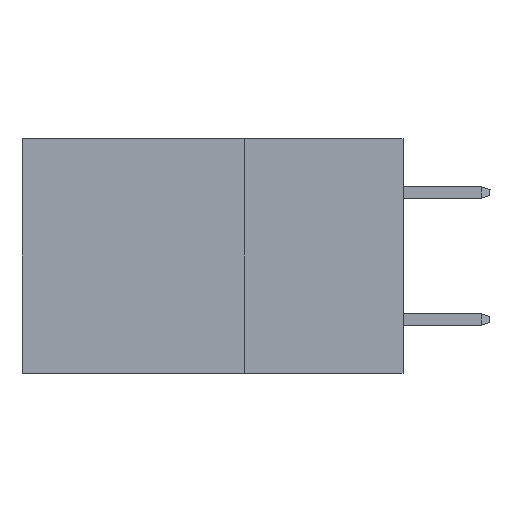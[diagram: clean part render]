
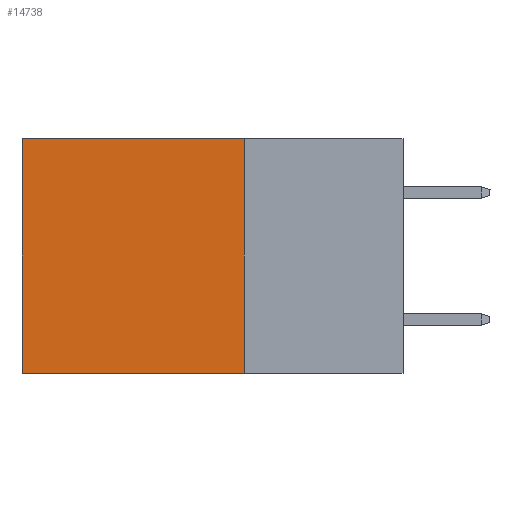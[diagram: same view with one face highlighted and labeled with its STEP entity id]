
A CAD part, left-side view. The second image highlights one B-rep face of the part: STEP entity #14738.
In plain terms, the highlighted planar face has unit normal (-1, 0, 0).
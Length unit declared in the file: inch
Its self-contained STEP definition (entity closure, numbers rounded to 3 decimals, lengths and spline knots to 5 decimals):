
#822 = EDGE_CURVE ( 'NONE', #19468, #3064, #5170, .T. ) ;
#952 = VECTOR ( 'NONE', #3561, 39.37008 ) ;
#962 = LINE ( 'NONE', #1295, #8657 ) ;
#1129 = VECTOR ( 'NONE', #20155, 39.37008 ) ;
#1295 = CARTESIAN_POINT ( 'NONE',  ( 0.2875, 0.25, 0. ) ) ;
#2134 = FACE_OUTER_BOUND ( 'NONE', #3882, .T. ) ;
#2595 = EDGE_CURVE ( 'NONE', #9917, #3064, #3316, .T. ) ;
#3039 = ORIENTED_EDGE ( 'NONE', *, *, #822, .F. ) ;
#3064 = VERTEX_POINT ( 'NONE', #18449 ) ;
#3134 = ORIENTED_EDGE ( 'NONE', *, *, #6986, .F. ) ;
#3316 = LINE ( 'NONE', #16810, #21057 ) ;
#3561 = DIRECTION ( 'NONE',  ( 0., 1., 0. ) ) ;
#3863 = DIRECTION ( 'NONE',  ( 0., 0., -1. ) ) ;
#3882 = EDGE_LOOP ( 'NONE', ( #5648, #3039, #3134, #20205 ) ) ;
#4609 = DIRECTION ( 'NONE',  ( 0., 0., -1. ) ) ;
#5120 = VERTEX_POINT ( 'NONE', #21756 ) ;
#5170 = LINE ( 'NONE', #17511, #952 ) ;
#5648 = ORIENTED_EDGE ( 'NONE', *, *, #2595, .T. ) ;
#6986 = EDGE_CURVE ( 'NONE', #5120, #19468, #962, .T. ) ;
#7045 = DIRECTION ( 'NONE',  ( 1., 0., 0. ) ) ;
#7315 = CARTESIAN_POINT ( 'NONE',  ( 0.2875, 0.6, 0. ) ) ;
#7955 = LINE ( 'NONE', #14931, #1129 ) ;
#8657 = VECTOR ( 'NONE', #4609, 39.37008 ) ;
#9917 = VERTEX_POINT ( 'NONE', #7315 ) ;
#10495 = PLANE ( 'NONE',  #18061 ) ;
#12256 = CARTESIAN_POINT ( 'NONE',  ( 0.2875, 0.25, -0.37 ) ) ;
#14477 = CARTESIAN_POINT ( 'NONE',  ( 0.2875, 0.25, 0. ) ) ;
#14738 = ADVANCED_FACE ( 'NONE', ( #2134 ), #10495, .F. ) ;
#14931 = CARTESIAN_POINT ( 'NONE',  ( 0.2875, 0.25, 0. ) ) ;
#16196 = DIRECTION ( 'NONE',  ( 0., 0., -1. ) ) ;
#16810 = CARTESIAN_POINT ( 'NONE',  ( 0.2875, 0.6, 0. ) ) ;
#17511 = CARTESIAN_POINT ( 'NONE',  ( 0.2875, 0.25, -0.37 ) ) ;
#18061 = AXIS2_PLACEMENT_3D ( 'NONE', #14477, #7045, #16196 ) ;
#18449 = CARTESIAN_POINT ( 'NONE',  ( 0.2875, 0.6, -0.37 ) ) ;
#19468 = VERTEX_POINT ( 'NONE', #12256 ) ;
#20155 = DIRECTION ( 'NONE',  ( 0., 1., 0. ) ) ;
#20205 = ORIENTED_EDGE ( 'NONE', *, *, #22276, .T. ) ;
#21057 = VECTOR ( 'NONE', #3863, 39.37008 ) ;
#21756 = CARTESIAN_POINT ( 'NONE',  ( 0.2875, 0.25, 0. ) ) ;
#22276 = EDGE_CURVE ( 'NONE', #5120, #9917, #7955, .T. ) ;
